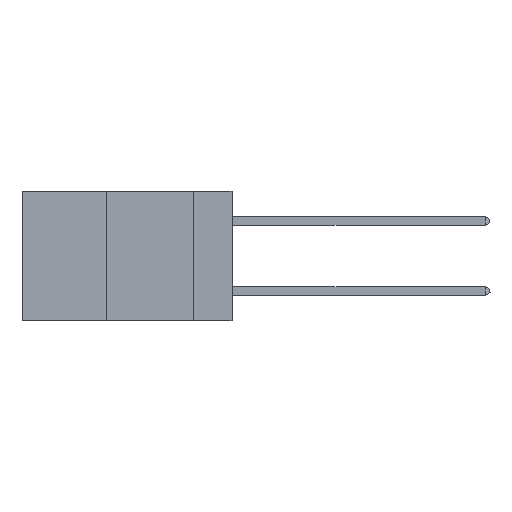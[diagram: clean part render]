
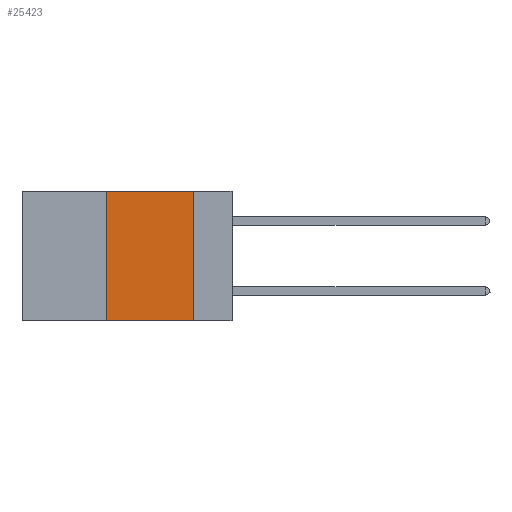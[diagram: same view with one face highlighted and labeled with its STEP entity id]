
A CAD part, left-side view. The second image highlights one B-rep face of the part: STEP entity #25423.
In plain terms, the highlighted planar face has unit normal (-1, 0, 0).
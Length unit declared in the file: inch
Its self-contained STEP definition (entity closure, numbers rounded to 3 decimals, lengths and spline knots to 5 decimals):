
#428 = VERTEX_POINT ( 'NONE', #5689 ) ;
#1547 = DIRECTION ( 'NONE',  ( 1., 0., 0. ) ) ;
#1596 = DIRECTION ( 'NONE',  ( 0., 0., -1. ) ) ;
#2420 = VECTOR ( 'NONE', #1596, 39.37008 ) ;
#2543 = VECTOR ( 'NONE', #19554, 39.37008 ) ;
#3876 = VERTEX_POINT ( 'NONE', #30654 ) ;
#4178 = LINE ( 'NONE', #10221, #26799 ) ;
#4395 = CARTESIAN_POINT ( 'NONE',  ( 0., 0.11, 0. ) ) ;
#4412 = FACE_OUTER_BOUND ( 'NONE', #4687, .T. ) ;
#4687 = EDGE_LOOP ( 'NONE', ( #19954, #20579, #8893, #25567 ) ) ;
#5689 = CARTESIAN_POINT ( 'NONE',  ( 0., 0.36, -0.37 ) ) ;
#5923 = CARTESIAN_POINT ( 'NONE',  ( 0., 0.11, 0. ) ) ;
#6535 = EDGE_CURVE ( 'NONE', #16720, #25038, #16747, .T. ) ;
#8893 = ORIENTED_EDGE ( 'NONE', *, *, #16139, .F. ) ;
#10221 = CARTESIAN_POINT ( 'NONE',  ( 0., 0.6, -0.37 ) ) ;
#11195 = EDGE_CURVE ( 'NONE', #428, #3876, #4178, .T. ) ;
#11581 = CARTESIAN_POINT ( 'NONE',  ( 0., 0.36, 0. ) ) ;
#11996 = PLANE ( 'NONE',  #22357 ) ;
#12104 = LINE ( 'NONE', #11581, #2543 ) ;
#14180 = EDGE_CURVE ( 'NONE', #25038, #3876, #27793, .T. ) ;
#16139 = EDGE_CURVE ( 'NONE', #428, #16720, #12104, .T. ) ;
#16310 = DIRECTION ( 'NONE',  ( 0., -1., 0. ) ) ;
#16720 = VERTEX_POINT ( 'NONE', #24555 ) ;
#16747 = LINE ( 'NONE', #26739, #30180 ) ;
#16760 = CARTESIAN_POINT ( 'NONE',  ( 0., 0.6, 0. ) ) ;
#19309 = DIRECTION ( 'NONE',  ( 0., 0., -1. ) ) ;
#19554 = DIRECTION ( 'NONE',  ( 0., 0., 1. ) ) ;
#19954 = ORIENTED_EDGE ( 'NONE', *, *, #14180, .F. ) ;
#20579 = ORIENTED_EDGE ( 'NONE', *, *, #6535, .F. ) ;
#22357 = AXIS2_PLACEMENT_3D ( 'NONE', #16760, #1547, #19309 ) ;
#23555 = DIRECTION ( 'NONE',  ( 0., -1., 0. ) ) ;
#24555 = CARTESIAN_POINT ( 'NONE',  ( 0., 0.36, 0. ) ) ;
#25038 = VERTEX_POINT ( 'NONE', #4395 ) ;
#25423 = ADVANCED_FACE ( 'NONE', ( #4412 ), #11996, .F. ) ;
#25567 = ORIENTED_EDGE ( 'NONE', *, *, #11195, .T. ) ;
#26739 = CARTESIAN_POINT ( 'NONE',  ( 0., 0.6, 0. ) ) ;
#26799 = VECTOR ( 'NONE', #23555, 39.37008 ) ;
#27793 = LINE ( 'NONE', #5923, #2420 ) ;
#30180 = VECTOR ( 'NONE', #16310, 39.37008 ) ;
#30654 = CARTESIAN_POINT ( 'NONE',  ( 0., 0.11, -0.37 ) ) ;
